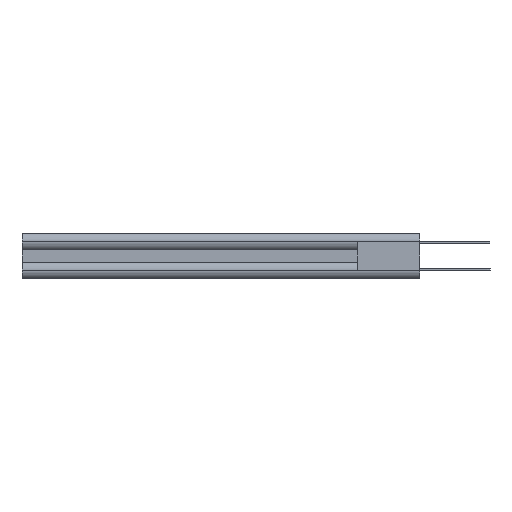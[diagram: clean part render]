
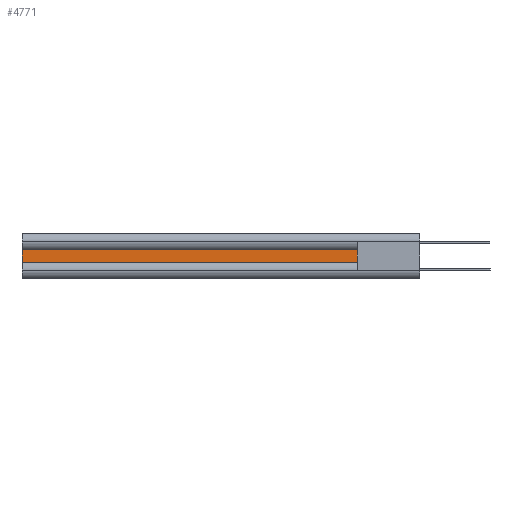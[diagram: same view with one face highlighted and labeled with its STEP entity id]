
A CAD part, left-side view. The second image highlights one B-rep face of the part: STEP entity #4771.
In plain terms, the highlighted planar face has unit normal (-1, 0, 0).
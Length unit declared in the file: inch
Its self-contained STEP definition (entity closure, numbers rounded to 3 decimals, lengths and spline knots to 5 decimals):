
#569 = CARTESIAN_POINT ( 'NONE',  ( 0.044, 0.473, -0.0465 ) ) ;
#1062 = DIRECTION ( 'NONE',  ( 0., 0., -1. ) ) ;
#1299 = VERTEX_POINT ( 'NONE', #11526 ) ;
#1525 = LINE ( 'NONE', #17621, #10201 ) ;
#1731 = EDGE_LOOP ( 'NONE', ( #11779, #4644, #10894, #9370 ) ) ;
#4644 = ORIENTED_EDGE ( 'NONE', *, *, #12619, .T. ) ;
#4771 = ADVANCED_FACE ( 'NONE', ( #16121 ), #13212, .F. ) ;
#4914 = VERTEX_POINT ( 'NONE', #13644 ) ;
#5817 = EDGE_CURVE ( 'NONE', #4914, #19048, #19912, .T. ) ;
#6485 = DIRECTION ( 'NONE',  ( 0., 0., -1. ) ) ;
#7853 = AXIS2_PLACEMENT_3D ( 'NONE', #14864, #16490, #6485 ) ;
#8485 = DIRECTION ( 'NONE',  ( 0., 1., 0. ) ) ;
#9370 = ORIENTED_EDGE ( 'NONE', *, *, #9619, .F. ) ;
#9619 = EDGE_CURVE ( 'NONE', #4914, #12589, #14900, .T. ) ;
#10201 = VECTOR ( 'NONE', #19258, 39.37008 ) ;
#10894 = ORIENTED_EDGE ( 'NONE', *, *, #12942, .F. ) ;
#10997 = CARTESIAN_POINT ( 'NONE',  ( 0.044, 0.37012, 0.0465 ) ) ;
#11155 = LINE ( 'NONE', #16754, #19348 ) ;
#11526 = CARTESIAN_POINT ( 'NONE',  ( 0.044, 3., -0.0465 ) ) ;
#11779 = ORIENTED_EDGE ( 'NONE', *, *, #5817, .T. ) ;
#12589 = VERTEX_POINT ( 'NONE', #569 ) ;
#12619 = EDGE_CURVE ( 'NONE', #19048, #1299, #1525, .T. ) ;
#12942 = EDGE_CURVE ( 'NONE', #12589, #1299, #11155, .T. ) ;
#13095 = CARTESIAN_POINT ( 'NONE',  ( 0.044, 0.473, -0.0465 ) ) ;
#13212 = PLANE ( 'NONE',  #7853 ) ;
#13644 = CARTESIAN_POINT ( 'NONE',  ( 0.044, 0.473, 0.0465 ) ) ;
#14542 = CARTESIAN_POINT ( 'NONE',  ( 0.044, 3., 0.0465 ) ) ;
#14864 = CARTESIAN_POINT ( 'NONE',  ( 0.044, 0.37012, -0.0465 ) ) ;
#14900 = LINE ( 'NONE', #13095, #19228 ) ;
#15069 = VECTOR ( 'NONE', #19231, 39.37008 ) ;
#16121 = FACE_OUTER_BOUND ( 'NONE', #1731, .T. ) ;
#16490 = DIRECTION ( 'NONE',  ( 1., 0., 0. ) ) ;
#16754 = CARTESIAN_POINT ( 'NONE',  ( 0.044, 0.37012, -0.0465 ) ) ;
#17621 = CARTESIAN_POINT ( 'NONE',  ( 0.044, 3., -0.0465 ) ) ;
#19048 = VERTEX_POINT ( 'NONE', #14542 ) ;
#19228 = VECTOR ( 'NONE', #1062, 39.37008 ) ;
#19231 = DIRECTION ( 'NONE',  ( 0., 1., 0. ) ) ;
#19258 = DIRECTION ( 'NONE',  ( 0., 0., -1. ) ) ;
#19348 = VECTOR ( 'NONE', #8485, 39.37008 ) ;
#19912 = LINE ( 'NONE', #10997, #15069 ) ;
